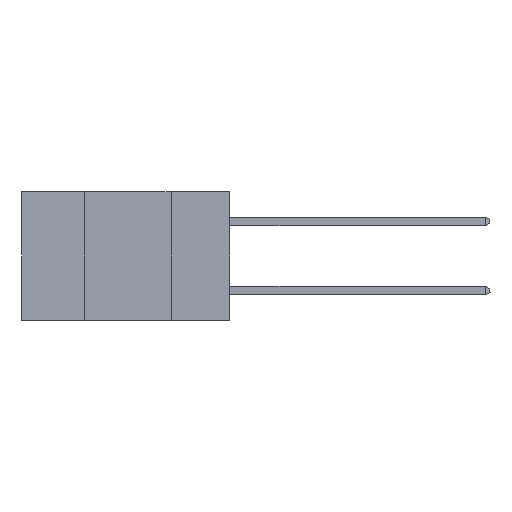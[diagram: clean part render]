
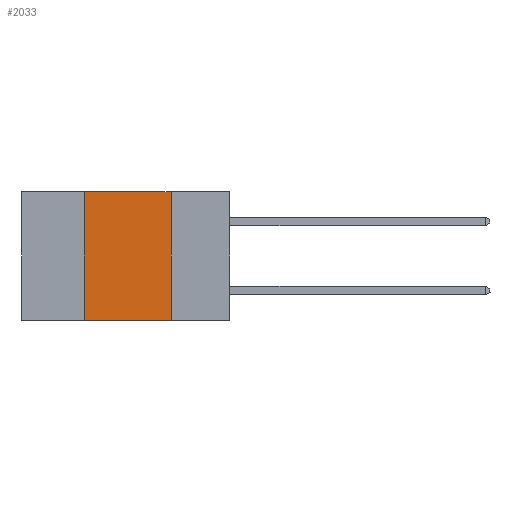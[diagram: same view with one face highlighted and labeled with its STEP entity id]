
A CAD part, left-side view. The second image highlights one B-rep face of the part: STEP entity #2033.
In plain terms, the highlighted planar face has unit normal (-1, 0, 0).
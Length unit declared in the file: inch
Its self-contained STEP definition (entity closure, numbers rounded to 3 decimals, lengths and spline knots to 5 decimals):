
#717 = LINE ( 'NONE', #6185, #1898 ) ;
#1898 = VECTOR ( 'NONE', #4747, 39.37008 ) ;
#2030 = DIRECTION ( 'NONE',  ( 1., 0., 0. ) ) ;
#2033 = ADVANCED_FACE ( 'NONE', ( #2502 ), #3750, .F. ) ;
#2142 = DIRECTION ( 'NONE',  ( 0., 0., -1. ) ) ;
#2502 = FACE_OUTER_BOUND ( 'NONE', #15843, .T. ) ;
#3175 = VERTEX_POINT ( 'NONE', #14511 ) ;
#3182 = CARTESIAN_POINT ( 'NONE',  ( 0., 0.6, -0.37 ) ) ;
#3750 = PLANE ( 'NONE',  #12531 ) ;
#3860 = EDGE_CURVE ( 'NONE', #10816, #13876, #18813, .T. ) ;
#4169 = CARTESIAN_POINT ( 'NONE',  ( 0., 0.42, -0.37 ) ) ;
#4747 = DIRECTION ( 'NONE',  ( 0., 0., 1. ) ) ;
#4875 = LINE ( 'NONE', #13461, #19560 ) ;
#4990 = ORIENTED_EDGE ( 'NONE', *, *, #3860, .T. ) ;
#6185 = CARTESIAN_POINT ( 'NONE',  ( 0., 0.42, 0. ) ) ;
#6597 = CARTESIAN_POINT ( 'NONE',  ( 0., 0.6, 0. ) ) ;
#6802 = VERTEX_POINT ( 'NONE', #16699 ) ;
#8276 = DIRECTION ( 'NONE',  ( 0., -1., 0. ) ) ;
#8551 = CARTESIAN_POINT ( 'NONE',  ( 0., 0.17, -0.37 ) ) ;
#9838 = CARTESIAN_POINT ( 'NONE',  ( 0., 0.6, 0. ) ) ;
#10313 = VECTOR ( 'NONE', #13233, 39.37008 ) ;
#10503 = DIRECTION ( 'NONE',  ( 0., 0., -1. ) ) ;
#10619 = VECTOR ( 'NONE', #8276, 39.37008 ) ;
#10816 = VERTEX_POINT ( 'NONE', #4169 ) ;
#11778 = LINE ( 'NONE', #9838, #10619 ) ;
#12167 = ORIENTED_EDGE ( 'NONE', *, *, #17499, .F. ) ;
#12531 = AXIS2_PLACEMENT_3D ( 'NONE', #6597, #2030, #2142 ) ;
#13053 = EDGE_CURVE ( 'NONE', #6802, #3175, #11778, .T. ) ;
#13233 = DIRECTION ( 'NONE',  ( 0., -1., 0. ) ) ;
#13275 = ORIENTED_EDGE ( 'NONE', *, *, #13943, .F. ) ;
#13461 = CARTESIAN_POINT ( 'NONE',  ( 0., 0.17, 0. ) ) ;
#13876 = VERTEX_POINT ( 'NONE', #8551 ) ;
#13943 = EDGE_CURVE ( 'NONE', #3175, #13876, #4875, .T. ) ;
#14511 = CARTESIAN_POINT ( 'NONE',  ( 0., 0.17, 0. ) ) ;
#15843 = EDGE_LOOP ( 'NONE', ( #13275, #17826, #12167, #4990 ) ) ;
#16699 = CARTESIAN_POINT ( 'NONE',  ( 0., 0.42, 0. ) ) ;
#17499 = EDGE_CURVE ( 'NONE', #10816, #6802, #717, .T. ) ;
#17826 = ORIENTED_EDGE ( 'NONE', *, *, #13053, .F. ) ;
#18813 = LINE ( 'NONE', #3182, #10313 ) ;
#19560 = VECTOR ( 'NONE', #10503, 39.37008 ) ;
